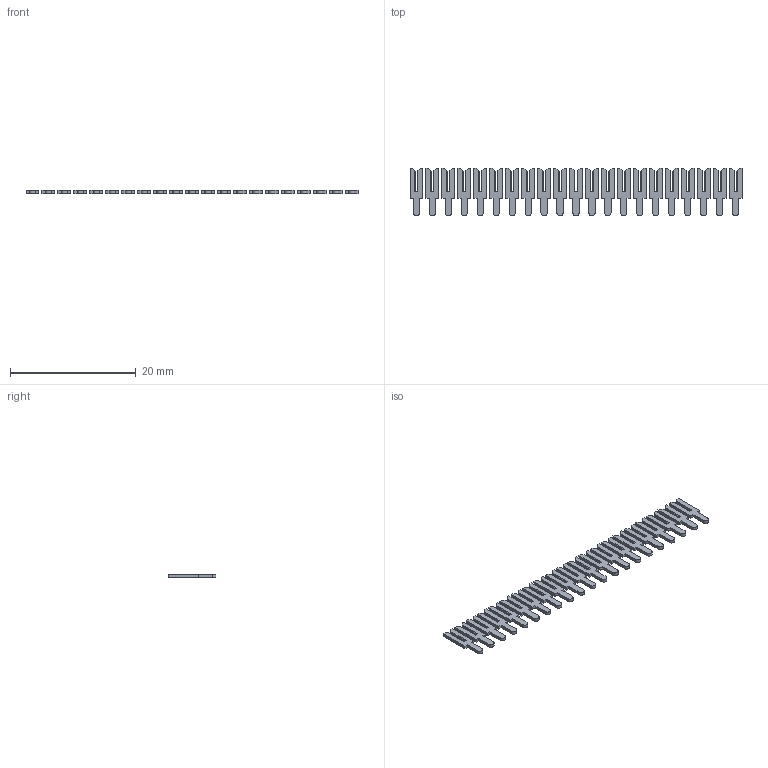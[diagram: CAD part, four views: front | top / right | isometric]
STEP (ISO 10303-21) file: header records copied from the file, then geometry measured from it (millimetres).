
FILE_DESCRIPTION (( 'STEP AP203' ), '1' );
FILE_NAME ('103-021-253-100.STEP', '2020-04-16T15:49:11', ( '' ), ( '' ), 'SwSTEP 2.0', 'SolidWorks 2016', '' );
FILE_SCHEMA (( 'CONFIG_CONTROL_DESIGN' ));
Length unit declared in the file: inch
Products named in the file (2): 103-021-253-100; 100-290-001_100-290-253
Assembly tree (21 placements, depth 2):
  103-021-253-100
    100-290-001_100-290-253  x21
Bounding box: 52.83 x 7.62 x 0.51 mm (x, y, z)
Volume: 115.9 mm3; surface area: 722.5 mm2
Topology: 21 solids, 21 shells, 420 faces, 1134 edges, 756 vertices
Faces by surface type: plane 399, cylinder 21
Entity records: 1460 total; most frequent: DIRECTION 144, CARTESIAN_POINT 134, ORIENTED_EDGE 108, EDGE_CURVE 54, DATE_AND_TIME 52, COORDINATED_UNIVERSAL_TIME_OFFSET 52, LOCAL_TIME 52, LINE 52
